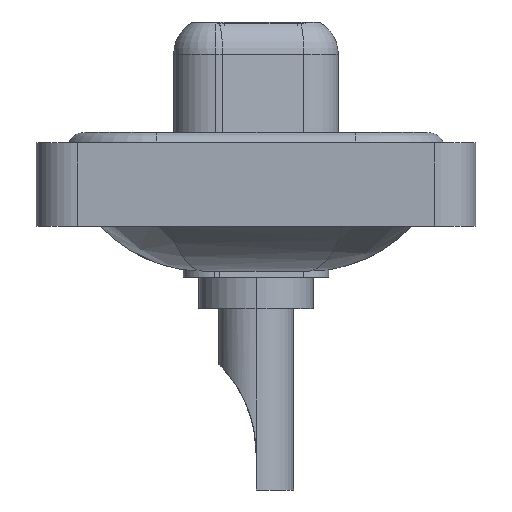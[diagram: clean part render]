
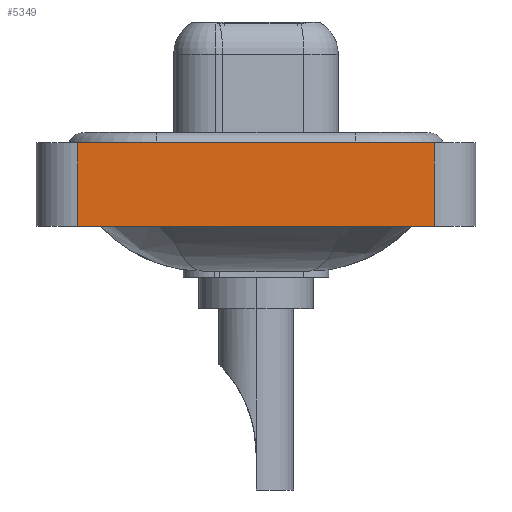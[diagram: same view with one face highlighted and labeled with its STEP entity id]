
A CAD part, left-side view. The second image highlights one B-rep face of the part: STEP entity #5349.
In plain terms, the highlighted planar face has unit normal (-1, 0, 0).
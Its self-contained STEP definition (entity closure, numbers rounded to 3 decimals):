
#248 = VERTEX_POINT ( 'NONE', #1047 ) ;
#394 = CARTESIAN_POINT ( 'NONE',  ( -7.25, -8.55, -3.6 ) ) ;
#724 = EDGE_LOOP ( 'NONE', ( #2091, #11657, #5861, #789 ) ) ;
#789 = ORIENTED_EDGE ( 'NONE', *, *, #15680, .T. ) ;
#1047 = CARTESIAN_POINT ( 'NONE',  ( -7.25, -8.55, 0.4 ) ) ;
#1350 = EDGE_CURVE ( 'NONE', #2875, #248, #13784, .T. ) ;
#1732 = FACE_OUTER_BOUND ( 'NONE', #724, .T. ) ;
#2091 = ORIENTED_EDGE ( 'NONE', *, *, #3977, .T. ) ;
#2813 = VERTEX_POINT ( 'NONE', #394 ) ;
#2875 = VERTEX_POINT ( 'NONE', #13449 ) ;
#3977 = EDGE_CURVE ( 'NONE', #2813, #248, #11346, .T. ) ;
#4262 = DIRECTION ( 'NONE',  ( 0., 0., 1. ) ) ;
#4378 = VECTOR ( 'NONE', #11177, 1000. ) ;
#4476 = VECTOR ( 'NONE', #11213, 1000. ) ;
#5349 = ADVANCED_FACE ( 'NONE', ( #1732 ), #16002, .T. ) ;
#5616 = EDGE_CURVE ( 'NONE', #12829, #2875, #12881, .T. ) ;
#5861 = ORIENTED_EDGE ( 'NONE', *, *, #5616, .F. ) ;
#7013 = AXIS2_PLACEMENT_3D ( 'NONE', #9728, #8167, #4262 ) ;
#7956 = CARTESIAN_POINT ( 'NONE',  ( -7.25, 8.55, -3.6 ) ) ;
#8167 = DIRECTION ( 'NONE',  ( -1., 0., 0. ) ) ;
#8272 = VECTOR ( 'NONE', #12972, 1000. ) ;
#9161 = CARTESIAN_POINT ( 'NONE',  ( -7.25, -8.55, -3.6 ) ) ;
#9728 = CARTESIAN_POINT ( 'NONE',  ( -7.25, -8.55, -3.6 ) ) ;
#10541 = VECTOR ( 'NONE', #14153, 1000. ) ;
#11177 = DIRECTION ( 'NONE',  ( 0., 0., 1. ) ) ;
#11213 = DIRECTION ( 'NONE',  ( 0., -1., 0. ) ) ;
#11346 = LINE ( 'NONE', #16418, #4378 ) ;
#11657 = ORIENTED_EDGE ( 'NONE', *, *, #1350, .F. ) ;
#11745 = LINE ( 'NONE', #9161, #10541 ) ;
#12829 = VERTEX_POINT ( 'NONE', #7956 ) ;
#12881 = LINE ( 'NONE', #13136, #8272 ) ;
#12972 = DIRECTION ( 'NONE',  ( 0., 0., 1. ) ) ;
#13136 = CARTESIAN_POINT ( 'NONE',  ( -7.25, 8.55, -3.6 ) ) ;
#13449 = CARTESIAN_POINT ( 'NONE',  ( -7.25, 8.55, 0.4 ) ) ;
#13784 = LINE ( 'NONE', #16455, #4476 ) ;
#14153 = DIRECTION ( 'NONE',  ( 0., -1., 0. ) ) ;
#15680 = EDGE_CURVE ( 'NONE', #12829, #2813, #11745, .T. ) ;
#16002 = PLANE ( 'NONE',  #7013 ) ;
#16418 = CARTESIAN_POINT ( 'NONE',  ( -7.25, -8.55, -3.6 ) ) ;
#16455 = CARTESIAN_POINT ( 'NONE',  ( -7.25, -8.55, 0.4 ) ) ;
